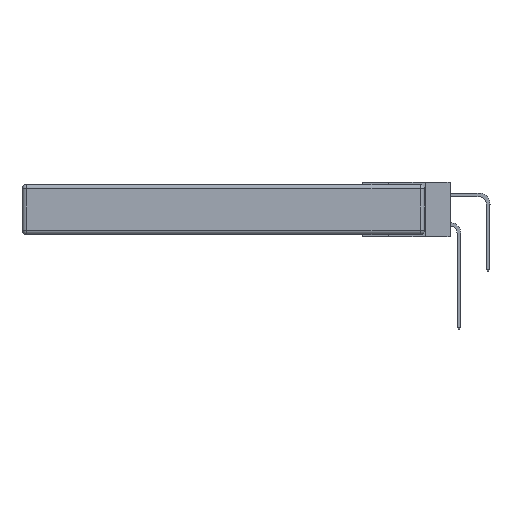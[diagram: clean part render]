
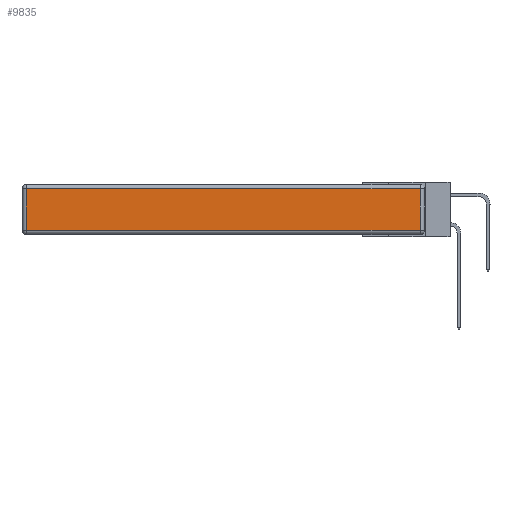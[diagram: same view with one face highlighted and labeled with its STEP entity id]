
A CAD part, left-side view. The second image highlights one B-rep face of the part: STEP entity #9835.
In plain terms, the highlighted planar face has unit normal (-1, 0, 0).
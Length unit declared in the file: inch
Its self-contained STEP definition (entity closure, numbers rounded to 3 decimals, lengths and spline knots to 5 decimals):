
#186 = CARTESIAN_POINT ( 'NONE',  ( 0., 2.72, -0.343 ) ) ;
#724 = FACE_OUTER_BOUND ( 'NONE', #5018, .T. ) ;
#772 = EDGE_CURVE ( 'NONE', #4513, #773, #1252, .T. ) ;
#773 = VERTEX_POINT ( 'NONE', #1319 ) ;
#1252 = LINE ( 'NONE', #8618, #13985 ) ;
#1319 = CARTESIAN_POINT ( 'NONE',  ( 0., 0.03, -0.313 ) ) ;
#1458 = DIRECTION ( 'NONE',  ( -1., 0., 0. ) ) ;
#2813 = CARTESIAN_POINT ( 'NONE',  ( 0., 0.03, -0.343 ) ) ;
#4041 = EDGE_CURVE ( 'NONE', #14099, #4513, #8251, .T. ) ;
#4513 = VERTEX_POINT ( 'NONE', #7584 ) ;
#4604 = ORIENTED_EDGE ( 'NONE', *, *, #772, .T. ) ;
#5018 = EDGE_LOOP ( 'NONE', ( #4604, #14360, #12006, #10849 ) ) ;
#5080 = VECTOR ( 'NONE', #6348, 39.37008 ) ;
#5273 = DIRECTION ( 'NONE',  ( 0., 0., 1. ) ) ;
#5278 = VECTOR ( 'NONE', #6971, 39.37008 ) ;
#5328 = EDGE_CURVE ( 'NONE', #773, #14702, #14952, .T. ) ;
#6348 = DIRECTION ( 'NONE',  ( 0., 0., 1. ) ) ;
#6971 = DIRECTION ( 'NONE',  ( 0., 1., 0. ) ) ;
#7340 = DIRECTION ( 'NONE',  ( 0., 0., -1. ) ) ;
#7584 = CARTESIAN_POINT ( 'NONE',  ( 0., 2.72, -0.313 ) ) ;
#8049 = CARTESIAN_POINT ( 'NONE',  ( 0., 0.03, -0.03 ) ) ;
#8251 = LINE ( 'NONE', #186, #10236 ) ;
#8618 = CARTESIAN_POINT ( 'NONE',  ( 0., 0., -0.313 ) ) ;
#8807 = CARTESIAN_POINT ( 'NONE',  ( 0., 0., -0.343 ) ) ;
#9835 = ADVANCED_FACE ( 'NONE', ( #724 ), #11283, .T. ) ;
#10115 = DIRECTION ( 'NONE',  ( 0., -1., 0. ) ) ;
#10236 = VECTOR ( 'NONE', #7340, 39.37008 ) ;
#10849 = ORIENTED_EDGE ( 'NONE', *, *, #4041, .T. ) ;
#11283 = PLANE ( 'NONE',  #12948 ) ;
#12006 = ORIENTED_EDGE ( 'NONE', *, *, #15838, .T. ) ;
#12948 = AXIS2_PLACEMENT_3D ( 'NONE', #8807, #1458, #5273 ) ;
#13985 = VECTOR ( 'NONE', #10115, 39.37008 ) ;
#14099 = VERTEX_POINT ( 'NONE', #15867 ) ;
#14360 = ORIENTED_EDGE ( 'NONE', *, *, #5328, .T. ) ;
#14381 = CARTESIAN_POINT ( 'NONE',  ( 0., 2.75, -0.03 ) ) ;
#14702 = VERTEX_POINT ( 'NONE', #8049 ) ;
#14952 = LINE ( 'NONE', #2813, #5080 ) ;
#15148 = LINE ( 'NONE', #14381, #5278 ) ;
#15838 = EDGE_CURVE ( 'NONE', #14702, #14099, #15148, .T. ) ;
#15867 = CARTESIAN_POINT ( 'NONE',  ( 0., 2.72, -0.03 ) ) ;
